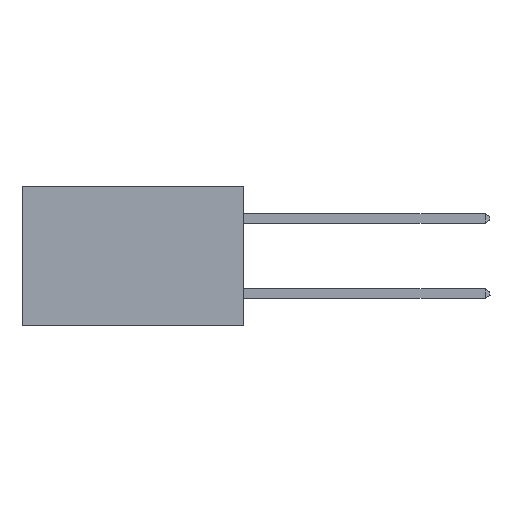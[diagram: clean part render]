
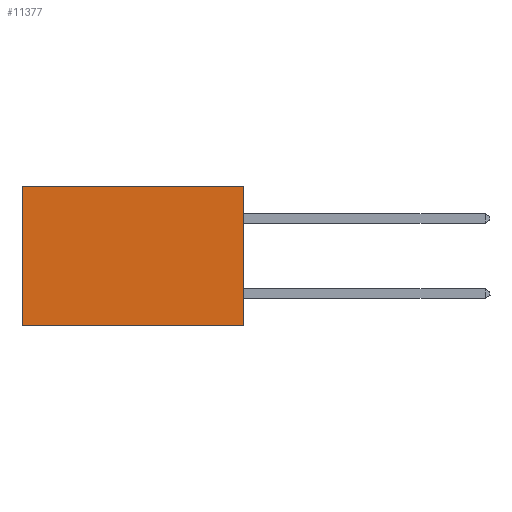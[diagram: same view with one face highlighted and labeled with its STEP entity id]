
A CAD part, left-side view. The second image highlights one B-rep face of the part: STEP entity #11377.
In plain terms, the highlighted planar face has unit normal (-1, 0, 0).
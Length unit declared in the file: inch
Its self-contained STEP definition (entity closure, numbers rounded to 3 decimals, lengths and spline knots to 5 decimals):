
#645 = VERTEX_POINT ( 'NONE', #2624 ) ;
#1433 = DIRECTION ( 'NONE',  ( 0., 0., -1. ) ) ;
#2470 = EDGE_CURVE ( 'NONE', #11348, #7413, #24049, .T. ) ;
#2624 = CARTESIAN_POINT ( 'NONE',  ( 0.277, 0.59, -0.37 ) ) ;
#4044 = CARTESIAN_POINT ( 'NONE',  ( 0.277, 0., 0. ) ) ;
#4135 = DIRECTION ( 'NONE',  ( 1., 0., 0. ) ) ;
#6039 = LINE ( 'NONE', #13547, #18136 ) ;
#6694 = CARTESIAN_POINT ( 'NONE',  ( 0.277, 0., 0. ) ) ;
#6917 = DIRECTION ( 'NONE',  ( 0., 1., 0. ) ) ;
#6999 = EDGE_CURVE ( 'NONE', #11348, #11727, #6039, .T. ) ;
#7116 = LINE ( 'NONE', #23918, #13522 ) ;
#7199 = ORIENTED_EDGE ( 'NONE', *, *, #2470, .T. ) ;
#7413 = VERTEX_POINT ( 'NONE', #7848 ) ;
#7821 = ORIENTED_EDGE ( 'NONE', *, *, #21257, .T. ) ;
#7848 = CARTESIAN_POINT ( 'NONE',  ( 0.277, 0.59, 0. ) ) ;
#9247 = EDGE_LOOP ( 'NONE', ( #7821, #23267, #25746, #7199 ) ) ;
#11348 = VERTEX_POINT ( 'NONE', #4044 ) ;
#11377 = ADVANCED_FACE ( 'NONE', ( #13327 ), #18655, .F. ) ;
#11727 = VERTEX_POINT ( 'NONE', #19872 ) ;
#13327 = FACE_OUTER_BOUND ( 'NONE', #9247, .T. ) ;
#13516 = VECTOR ( 'NONE', #6917, 39.37008 ) ;
#13522 = VECTOR ( 'NONE', #16764, 39.37008 ) ;
#13547 = CARTESIAN_POINT ( 'NONE',  ( 0.277, 0., -0.37 ) ) ;
#16224 = CARTESIAN_POINT ( 'NONE',  ( 0.277, 0., -0.37 ) ) ;
#16764 = DIRECTION ( 'NONE',  ( 0., 0., -1. ) ) ;
#17388 = CARTESIAN_POINT ( 'NONE',  ( 0.277, 0., -0.37 ) ) ;
#18136 = VECTOR ( 'NONE', #1433, 39.37008 ) ;
#18655 = PLANE ( 'NONE',  #20547 ) ;
#19773 = DIRECTION ( 'NONE',  ( 0., 1., 0. ) ) ;
#19872 = CARTESIAN_POINT ( 'NONE',  ( 0.277, 0., -0.37 ) ) ;
#20547 = AXIS2_PLACEMENT_3D ( 'NONE', #16224, #4135, #21052 ) ;
#21052 = DIRECTION ( 'NONE',  ( 0., 0., -1. ) ) ;
#21257 = EDGE_CURVE ( 'NONE', #7413, #645, #7116, .T. ) ;
#23267 = ORIENTED_EDGE ( 'NONE', *, *, #27829, .F. ) ;
#23918 = CARTESIAN_POINT ( 'NONE',  ( 0.277, 0.59, -0.37 ) ) ;
#24049 = LINE ( 'NONE', #6694, #13516 ) ;
#25746 = ORIENTED_EDGE ( 'NONE', *, *, #6999, .F. ) ;
#27829 = EDGE_CURVE ( 'NONE', #11727, #645, #29805, .T. ) ;
#29047 = VECTOR ( 'NONE', #19773, 39.37008 ) ;
#29805 = LINE ( 'NONE', #17388, #29047 ) ;
